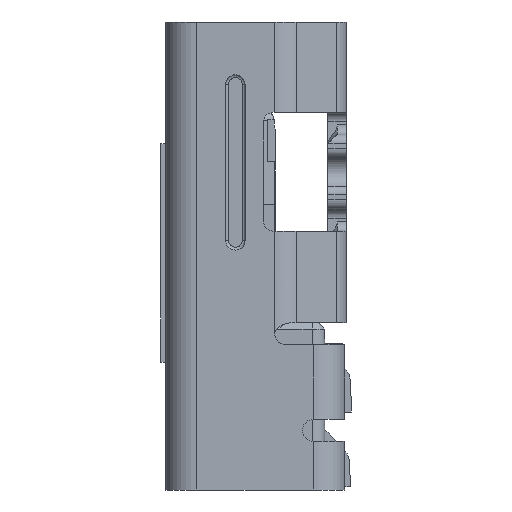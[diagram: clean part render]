
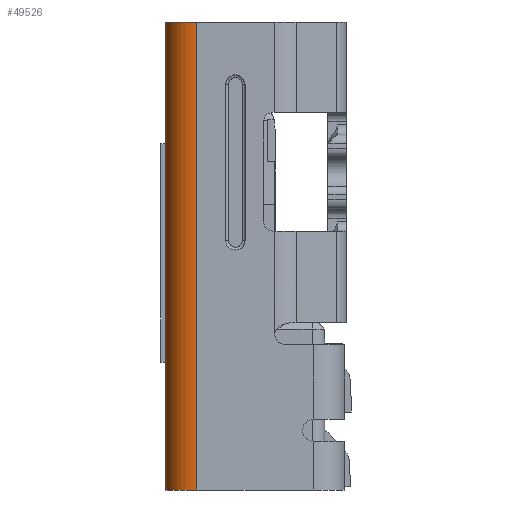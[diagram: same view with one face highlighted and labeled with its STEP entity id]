
A CAD part, left-side view. The second image highlights one B-rep face of the part: STEP entity #49526.
In plain terms, the highlighted cylindrical face has radius 0.5 mm (diameter 1 mm), a partial arc.
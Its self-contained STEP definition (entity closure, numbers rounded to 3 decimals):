
#298 = DIRECTION ( 'NONE',  ( -1., 0., 0. ) ) ;
#1306 = CARTESIAN_POINT ( 'NONE',  ( -2.75, 0., -7.5 ) ) ;
#1889 = EDGE_CURVE ( 'NONE', #40120, #27595, #62384, .T. ) ;
#2742 = AXIS2_PLACEMENT_3D ( 'NONE', #29285, #53219, #298 ) ;
#3656 = CARTESIAN_POINT ( 'NONE',  ( -3.25, -0.5, -2.5 ) ) ;
#6001 = ORIENTED_EDGE ( 'NONE', *, *, #1889, .F. ) ;
#11308 = FACE_OUTER_BOUND ( 'NONE', #11603, .T. ) ;
#11603 = EDGE_LOOP ( 'NONE', ( #6001, #61970, #37912, #58505 ) ) ;
#13778 = CARTESIAN_POINT ( 'NONE',  ( -3.25, -0.5, -7.5 ) ) ;
#19720 = AXIS2_PLACEMENT_3D ( 'NONE', #36785, #32036, #59546 ) ;
#27595 = VERTEX_POINT ( 'NONE', #42795 ) ;
#28348 = DIRECTION ( 'NONE',  ( 0., 0., 1. ) ) ;
#29285 = CARTESIAN_POINT ( 'NONE',  ( -2.75, -0.5, -7.5 ) ) ;
#31240 = VERTEX_POINT ( 'NONE', #49890 ) ;
#32036 = DIRECTION ( 'NONE',  ( 0., 0., 1. ) ) ;
#32379 = B_SPLINE_CURVE_WITH_KNOTS ( 'NONE', 3,
 ( #13778, #46863, #3656, #47788 ),
 .UNSPECIFIED., .F., .F.,
 ( 4, 4 ),
 ( 0., 1. ),
 .UNSPECIFIED. ) ;
#33137 = DIRECTION ( 'NONE',  ( -1., 0., 0. ) ) ;
#34935 = AXIS2_PLACEMENT_3D ( 'NONE', #46714, #37893, #33137 ) ;
#36785 = CARTESIAN_POINT ( 'NONE',  ( -2.75, -0.5, -7.5 ) ) ;
#36835 = CIRCLE ( 'NONE', #19720, 0.5 ) ;
#37893 = DIRECTION ( 'NONE',  ( 0., 0., -1. ) ) ;
#37912 = ORIENTED_EDGE ( 'NONE', *, *, #44089, .T. ) ;
#37967 = CIRCLE ( 'NONE', #34935, 0.5 ) ;
#38733 = CARTESIAN_POINT ( 'NONE',  ( -3.25, -0.5, 0. ) ) ;
#40120 = VERTEX_POINT ( 'NONE', #1306 ) ;
#42795 = CARTESIAN_POINT ( 'NONE',  ( -2.75, 0., 0. ) ) ;
#44089 = EDGE_CURVE ( 'NONE', #31240, #62139, #32379, .T. ) ;
#46714 = CARTESIAN_POINT ( 'NONE',  ( -2.75, -0.5, 0. ) ) ;
#46863 = CARTESIAN_POINT ( 'NONE',  ( -3.25, -0.5, -5. ) ) ;
#47691 = EDGE_CURVE ( 'NONE', #40120, #31240, #36835, .T. ) ;
#47788 = CARTESIAN_POINT ( 'NONE',  ( -3.25, -0.5, 0. ) ) ;
#48355 = EDGE_CURVE ( 'NONE', #62139, #27595, #37967, .T. ) ;
#49526 = ADVANCED_FACE ( 'NONE', ( #11308 ), #58583, .T. ) ;
#49890 = CARTESIAN_POINT ( 'NONE',  ( -3.25, -0.5, -7.5 ) ) ;
#52288 = CARTESIAN_POINT ( 'NONE',  ( -2.75, 0., 0. ) ) ;
#53219 = DIRECTION ( 'NONE',  ( 0., 0., -1. ) ) ;
#58505 = ORIENTED_EDGE ( 'NONE', *, *, #48355, .T. ) ;
#58583 = CYLINDRICAL_SURFACE ( 'NONE', #2742, 0.5 ) ;
#59546 = DIRECTION ( 'NONE',  ( -1., 0., 0. ) ) ;
#61248 = VECTOR ( 'NONE', #28348, 1000. ) ;
#61970 = ORIENTED_EDGE ( 'NONE', *, *, #47691, .T. ) ;
#62139 = VERTEX_POINT ( 'NONE', #38733 ) ;
#62384 = LINE ( 'NONE', #52288, #61248 ) ;
